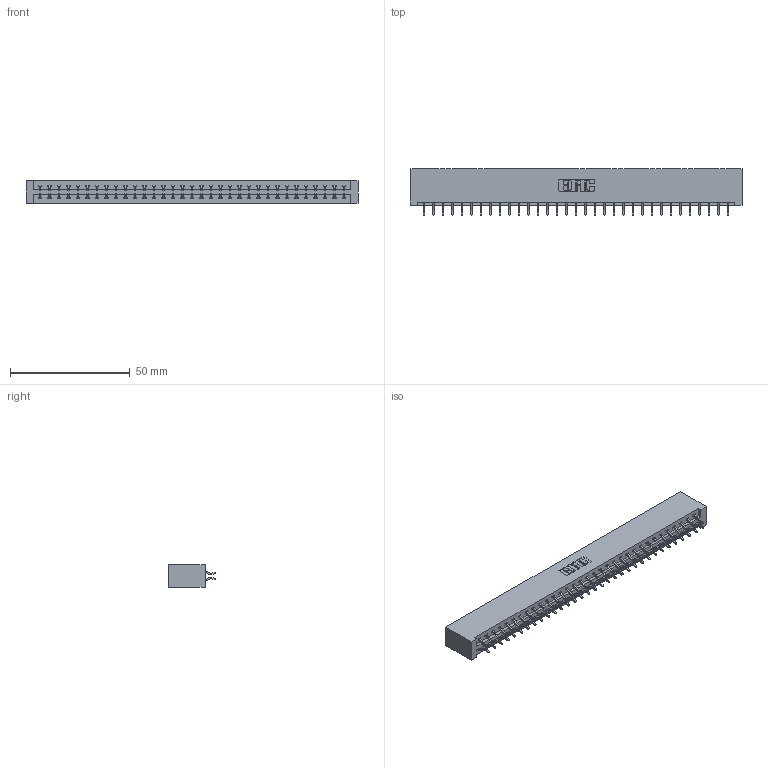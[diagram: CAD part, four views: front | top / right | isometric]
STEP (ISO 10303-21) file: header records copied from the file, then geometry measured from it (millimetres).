
FILE_DESCRIPTION (( 'STEP AP203' ), '1' );
FILE_NAME ('337-066-556-201.STEP', '2018-08-11T08:29:33', ( '' ), ( '' ), 'SwSTEP 2.0', 'SolidWorks 2016', '' );
FILE_SCHEMA (( 'CONFIG_CONTROL_DESIGN' ));
Length unit declared in the file: inch
Products named in the file (3): 337-066-556-201; 337 Part_No Mounting Lugs; 345-292-001_556 Tail
Assembly tree (67 placements, depth 2):
  337-066-556-201
    337 Part_No Mounting Lugs
    345-292-001_556 Tail  x66
Bounding box: 138.63 x 19.57 x 9.4 mm (x, y, z)
Volume: 15248.6 mm3; surface area: 17137.6 mm2
Topology: 67 solids, 67 shells, 4066 faces, 12101 edges, 7978 vertices
Faces by surface type: plane 2838, cylinder 1228
Entity records: 26693 total; most frequent: CARTESIAN_POINT 4518, ORIENTED_EDGE 4442, DIRECTION 3841, EDGE_CURVE 2221, VECTOR 2093, LINE 2093, VERTEX_POINT 1478, AXIS2_PLACEMENT_3D 874
